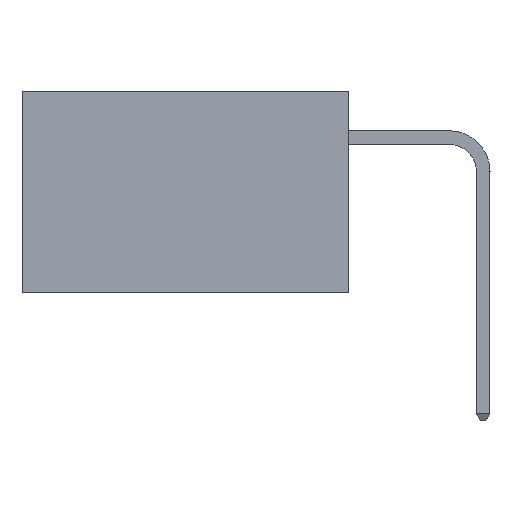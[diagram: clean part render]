
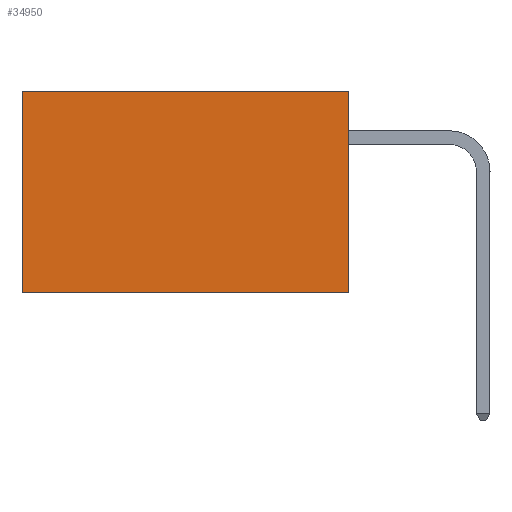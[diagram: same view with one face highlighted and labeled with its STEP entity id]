
A CAD part, left-side view. The second image highlights one B-rep face of the part: STEP entity #34950.
In plain terms, the highlighted planar face has unit normal (-1, 0, 0).
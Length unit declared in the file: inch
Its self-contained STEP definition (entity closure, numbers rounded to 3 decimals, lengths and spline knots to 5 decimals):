
#630 = ORIENTED_EDGE ( 'NONE', *, *, #16764, .F. ) ;
#926 = VECTOR ( 'NONE', #23159, 39.37008 ) ;
#967 = DIRECTION ( 'NONE',  ( 0., 0., -1. ) ) ;
#1406 = DIRECTION ( 'NONE',  ( 1., 0., 0. ) ) ;
#2679 = VERTEX_POINT ( 'NONE', #22490 ) ;
#3551 = CARTESIAN_POINT ( 'NONE',  ( 0.2875, 0., 0. ) ) ;
#4375 = VERTEX_POINT ( 'NONE', #31647 ) ;
#4984 = CARTESIAN_POINT ( 'NONE',  ( 0.2875, 0., 0. ) ) ;
#7868 = LINE ( 'NONE', #17196, #926 ) ;
#9765 = EDGE_CURVE ( 'NONE', #18000, #2679, #37669, .T. ) ;
#12163 = AXIS2_PLACEMENT_3D ( 'NONE', #16138, #1406, #22114 ) ;
#16138 = CARTESIAN_POINT ( 'NONE',  ( 0.2875, 0., 0. ) ) ;
#16455 = EDGE_CURVE ( 'NONE', #18000, #4375, #34664, .T. ) ;
#16764 = EDGE_CURVE ( 'NONE', #4375, #34058, #7868, .T. ) ;
#17196 = CARTESIAN_POINT ( 'NONE',  ( 0.2875, 0., -0.37 ) ) ;
#17408 = ORIENTED_EDGE ( 'NONE', *, *, #9765, .T. ) ;
#18000 = VERTEX_POINT ( 'NONE', #4984 ) ;
#18045 = EDGE_LOOP ( 'NONE', ( #34601, #630, #33106, #17408 ) ) ;
#18663 = CARTESIAN_POINT ( 'NONE',  ( 0.2875, 0.6, 0. ) ) ;
#21775 = CARTESIAN_POINT ( 'NONE',  ( 0.2875, 0., 0. ) ) ;
#22114 = DIRECTION ( 'NONE',  ( 0., 0., -1. ) ) ;
#22490 = CARTESIAN_POINT ( 'NONE',  ( 0.2875, 0.6, 0. ) ) ;
#23159 = DIRECTION ( 'NONE',  ( 0., 1., 0. ) ) ;
#23358 = FACE_OUTER_BOUND ( 'NONE', #18045, .T. ) ;
#25916 = VECTOR ( 'NONE', #30149, 39.37008 ) ;
#29886 = VECTOR ( 'NONE', #33623, 39.37008 ) ;
#29936 = EDGE_CURVE ( 'NONE', #2679, #34058, #38124, .T. ) ;
#30149 = DIRECTION ( 'NONE',  ( 0., 0., -1. ) ) ;
#31271 = VECTOR ( 'NONE', #967, 39.37008 ) ;
#31647 = CARTESIAN_POINT ( 'NONE',  ( 0.2875, 0., -0.37 ) ) ;
#33106 = ORIENTED_EDGE ( 'NONE', *, *, #16455, .F. ) ;
#33623 = DIRECTION ( 'NONE',  ( 0., 1., 0. ) ) ;
#34058 = VERTEX_POINT ( 'NONE', #34908 ) ;
#34601 = ORIENTED_EDGE ( 'NONE', *, *, #29936, .T. ) ;
#34664 = LINE ( 'NONE', #3551, #25916 ) ;
#34908 = CARTESIAN_POINT ( 'NONE',  ( 0.2875, 0.6, -0.37 ) ) ;
#34950 = ADVANCED_FACE ( 'NONE', ( #23358 ), #36770, .F. ) ;
#36770 = PLANE ( 'NONE',  #12163 ) ;
#37669 = LINE ( 'NONE', #21775, #29886 ) ;
#38124 = LINE ( 'NONE', #18663, #31271 ) ;
